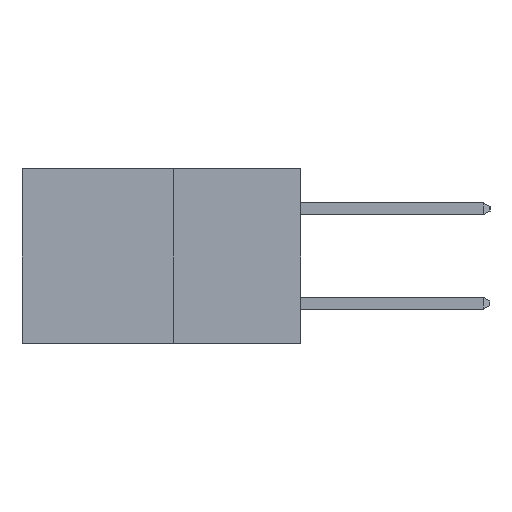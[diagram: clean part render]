
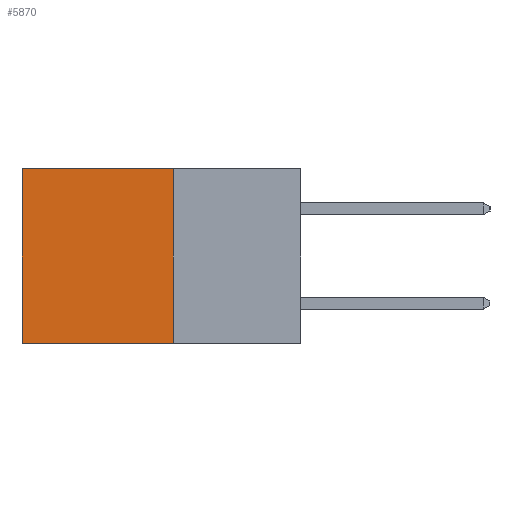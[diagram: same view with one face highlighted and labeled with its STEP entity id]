
A CAD part, left-side view. The second image highlights one B-rep face of the part: STEP entity #5870.
In plain terms, the highlighted planar face has unit normal (-1, 0, 0).
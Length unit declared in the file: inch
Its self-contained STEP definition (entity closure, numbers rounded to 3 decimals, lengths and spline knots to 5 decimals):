
#1699 = VECTOR ( 'NONE', #7649, 39.37008 ) ;
#2515 = VERTEX_POINT ( 'NONE', #19347 ) ;
#2844 = ORIENTED_EDGE ( 'NONE', *, *, #16345, .F. ) ;
#3538 = DIRECTION ( 'NONE',  ( 0., 1., 0. ) ) ;
#4084 = ORIENTED_EDGE ( 'NONE', *, *, #12780, .T. ) ;
#4550 = ORIENTED_EDGE ( 'NONE', *, *, #12468, .F. ) ;
#4783 = EDGE_LOOP ( 'NONE', ( #4084, #4550, #2844, #5982 ) ) ;
#5196 = CARTESIAN_POINT ( 'NONE',  ( 0.277, 0.59, 0. ) ) ;
#5300 = VERTEX_POINT ( 'NONE', #12842 ) ;
#5870 = ADVANCED_FACE ( 'NONE', ( #19387 ), #14638, .F. ) ;
#5982 = ORIENTED_EDGE ( 'NONE', *, *, #13474, .T. ) ;
#6019 = CARTESIAN_POINT ( 'NONE',  ( 0.277, 0.27, -0.37 ) ) ;
#6628 = VERTEX_POINT ( 'NONE', #5196 ) ;
#7459 = VECTOR ( 'NONE', #8968, 39.37008 ) ;
#7649 = DIRECTION ( 'NONE',  ( 0., 1., 0. ) ) ;
#8590 = CARTESIAN_POINT ( 'NONE',  ( 0.277, 0.59, -0.37 ) ) ;
#8634 = VECTOR ( 'NONE', #13180, 39.37008 ) ;
#8968 = DIRECTION ( 'NONE',  ( 0., 0., -1. ) ) ;
#10156 = VERTEX_POINT ( 'NONE', #8590 ) ;
#11766 = LINE ( 'NONE', #16849, #7459 ) ;
#12405 = LINE ( 'NONE', #13111, #8634 ) ;
#12468 = EDGE_CURVE ( 'NONE', #2515, #10156, #15640, .T. ) ;
#12780 = EDGE_CURVE ( 'NONE', #6628, #10156, #12405, .T. ) ;
#12842 = CARTESIAN_POINT ( 'NONE',  ( 0.277, 0.27, 0. ) ) ;
#13111 = CARTESIAN_POINT ( 'NONE',  ( 0.277, 0.59, -0.37 ) ) ;
#13180 = DIRECTION ( 'NONE',  ( 0., 0., -1. ) ) ;
#13250 = CARTESIAN_POINT ( 'NONE',  ( 0.277, 0.27, 0. ) ) ;
#13474 = EDGE_CURVE ( 'NONE', #5300, #6628, #19975, .T. ) ;
#14193 = AXIS2_PLACEMENT_3D ( 'NONE', #14572, #14526, #14519 ) ;
#14519 = DIRECTION ( 'NONE',  ( 0., 0., -1. ) ) ;
#14526 = DIRECTION ( 'NONE',  ( 1., 0., 0. ) ) ;
#14572 = CARTESIAN_POINT ( 'NONE',  ( 0.277, 0.27, -0.37 ) ) ;
#14638 = PLANE ( 'NONE',  #14193 ) ;
#15640 = LINE ( 'NONE', #6019, #1699 ) ;
#16345 = EDGE_CURVE ( 'NONE', #5300, #2515, #11766, .T. ) ;
#16786 = VECTOR ( 'NONE', #3538, 39.37008 ) ;
#16849 = CARTESIAN_POINT ( 'NONE',  ( 0.277, 0.27, -0.37 ) ) ;
#19347 = CARTESIAN_POINT ( 'NONE',  ( 0.277, 0.27, -0.37 ) ) ;
#19387 = FACE_OUTER_BOUND ( 'NONE', #4783, .T. ) ;
#19975 = LINE ( 'NONE', #13250, #16786 ) ;
